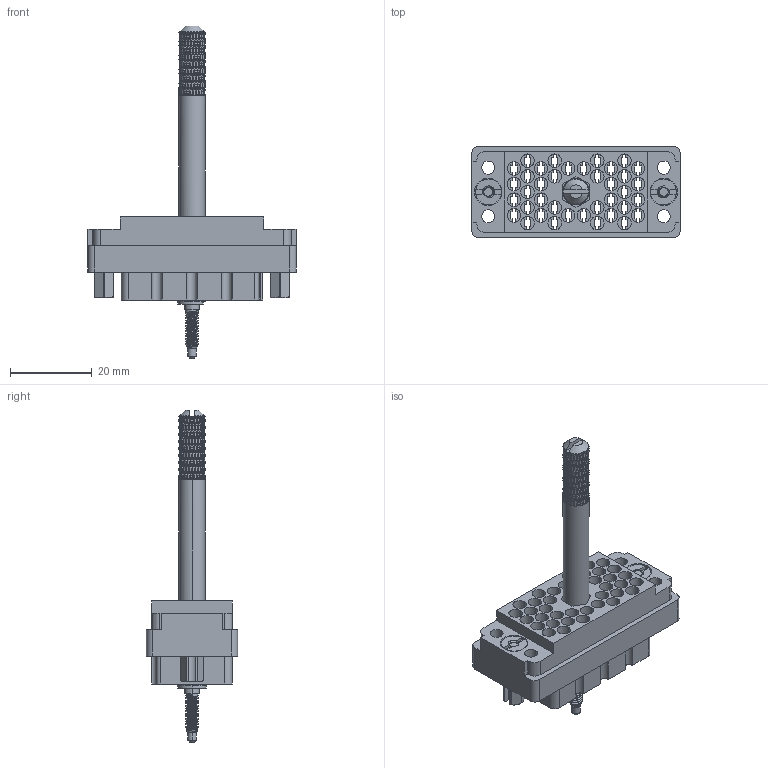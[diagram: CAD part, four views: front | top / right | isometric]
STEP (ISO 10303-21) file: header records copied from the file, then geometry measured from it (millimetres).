
FILE_DESCRIPTION (( 'STEP AP203' ), '1' );
FILE_NAME ('516-038-000-201.STEP', '2020-03-04T21:13:19', ( '' ), ( '' ), 'SwSTEP 2.0', 'SolidWorks 2016', '' );
FILE_SCHEMA (( 'CONFIG_CONTROL_DESIGN' ));
Length unit declared in the file: inch
Products named in the file (10): 516-250-038-111; 516-252-021-102_038; 516-251-035-100; 516-253-138-107; 516-221-038-102_039; Actuating Screw Assy 038-056; 516-038-000-201; 516-253-035-100; 516 Part Receptacle_038; 516-221-038-102_038
Assembly tree (11 placements, depth 3):
  516-038-000-201
    516 Part Receptacle_038
    516-252-021-102_038  x2
    516-221-038-102_038
    Actuating Screw Assy 038-056
      516-251-035-100
      516-253-035-100  x2
      516-253-138-107
      516-250-038-111
    516-221-038-102_039
Bounding box: 50.8 x 22.25 x 81.03 mm (x, y, z)
Volume: 13072.4 mm3; surface area: 17490 mm2
Topology: 10 solids, 10 shells, 2484 faces, 6150 edges, 3702 vertices
Faces by surface type: bspline 1034, plane 760, cylinder 638, cone 52
Entity records: 106324 total; most frequent: CARTESIAN_POINT 58853, ORIENTED_EDGE 12088, DIRECTION 7074, EDGE_CURVE 6044, VERTEX_POINT 3634, EDGE_LOOP 2564, ADVANCED_FACE 2447, FACE_OUTER_BOUND 2447
